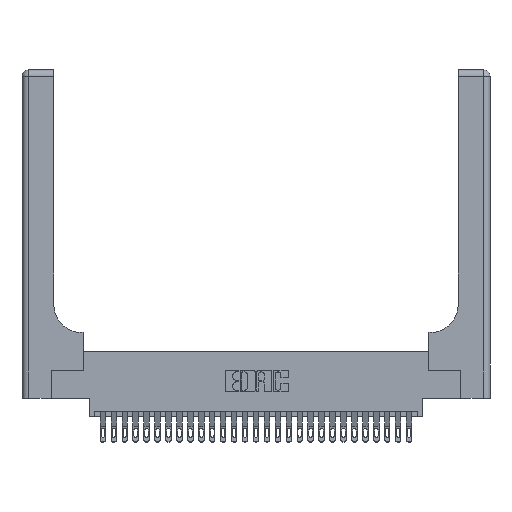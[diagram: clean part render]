
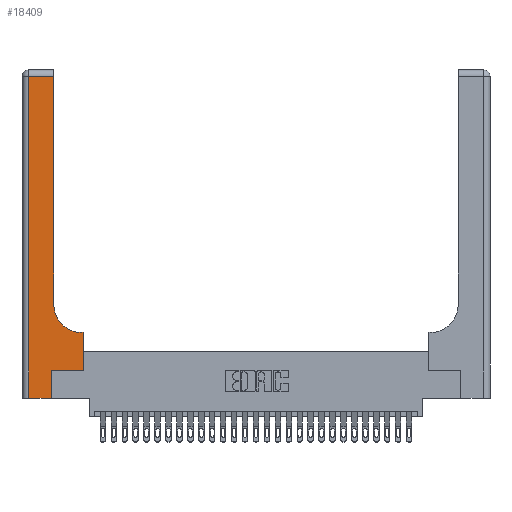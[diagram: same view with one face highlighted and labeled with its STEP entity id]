
A CAD part, top view. The second image highlights one B-rep face of the part: STEP entity #18409.
In plain terms, the highlighted planar face has unit normal (0, 0, 1).
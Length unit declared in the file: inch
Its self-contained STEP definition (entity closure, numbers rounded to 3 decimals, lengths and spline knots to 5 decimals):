
#286 = LINE ( 'NONE', #29369, #20678 ) ;
#316 = ORIENTED_EDGE ( 'NONE', *, *, #1846, .T. ) ;
#583 = LINE ( 'NONE', #9753, #21676 ) ;
#1080 = CARTESIAN_POINT ( 'NONE',  ( 0.5415, 0.6, 0.37 ) ) ;
#1422 = DIRECTION ( 'NONE',  ( 1., 0., 0. ) ) ;
#1766 = CARTESIAN_POINT ( 'NONE',  ( 0.2915, 0.85, 0.37 ) ) ;
#1846 = EDGE_CURVE ( 'NONE', #19101, #23608, #29240, .T. ) ;
#1951 = ORIENTED_EDGE ( 'NONE', *, *, #27881, .T. ) ;
#2306 = VERTEX_POINT ( 'NONE', #18966 ) ;
#2532 = DIRECTION ( 'NONE',  ( 0., 0., -1. ) ) ;
#3046 = DIRECTION ( 'NONE',  ( 0., 1., 0. ) ) ;
#3191 = VECTOR ( 'NONE', #5815, 39.37008 ) ;
#4720 = VECTOR ( 'NONE', #18654, 39.37008 ) ;
#4853 = VECTOR ( 'NONE', #23996, 39.37008 ) ;
#5710 = EDGE_CURVE ( 'NONE', #20794, #19314, #24332, .T. ) ;
#5815 = DIRECTION ( 'NONE',  ( -1., 0., 0. ) ) ;
#5923 = VERTEX_POINT ( 'NONE', #26721 ) ;
#5955 = ORIENTED_EDGE ( 'NONE', *, *, #25699, .T. ) ;
#6012 = DIRECTION ( 'NONE',  ( 0., -1., 0. ) ) ;
#6701 = CARTESIAN_POINT ( 'NONE',  ( 0., 0., 0.37 ) ) ;
#6888 = ORIENTED_EDGE ( 'NONE', *, *, #22023, .T. ) ;
#6964 = VECTOR ( 'NONE', #27529, 39.37008 ) ;
#8255 = CARTESIAN_POINT ( 'NONE',  ( 0.06, 3., 0.37 ) ) ;
#8374 = EDGE_CURVE ( 'NONE', #19314, #13760, #583, .T. ) ;
#9335 = VECTOR ( 'NONE', #27791, 39.37008 ) ;
#9753 = CARTESIAN_POINT ( 'NONE',  ( 0.2915, 3., 0.37 ) ) ;
#10920 = VERTEX_POINT ( 'NONE', #23585 ) ;
#12818 = CARTESIAN_POINT ( 'NONE',  ( 0.2915, 0.6, 0.37 ) ) ;
#13596 = LINE ( 'NONE', #8255, #25254 ) ;
#13760 = VERTEX_POINT ( 'NONE', #16475 ) ;
#13854 = VERTEX_POINT ( 'NONE', #25062 ) ;
#14559 = LINE ( 'NONE', #6701, #6964 ) ;
#16033 = ORIENTED_EDGE ( 'NONE', *, *, #28405, .T. ) ;
#16475 = CARTESIAN_POINT ( 'NONE',  ( 0.2915, 2.94, 0.37 ) ) ;
#16547 = CARTESIAN_POINT ( 'NONE',  ( 0.5585, 0.25, 0.37 ) ) ;
#16715 = ORIENTED_EDGE ( 'NONE', *, *, #5710, .T. ) ;
#17012 = FACE_OUTER_BOUND ( 'NONE', #23075, .T. ) ;
#17304 = LINE ( 'NONE', #12818, #3191 ) ;
#17725 = CARTESIAN_POINT ( 'NONE',  ( 0., 2.94, 0.37 ) ) ;
#17906 = CARTESIAN_POINT ( 'NONE',  ( 0.5415, 0.85, 0.37 ) ) ;
#18409 = ADVANCED_FACE ( 'NONE', ( #17012 ), #21567, .F. ) ;
#18654 = DIRECTION ( 'NONE',  ( 0., 1., 0. ) ) ;
#18966 = CARTESIAN_POINT ( 'NONE',  ( 0.5585, 0.6, 0.37 ) ) ;
#19101 = VERTEX_POINT ( 'NONE', #19799 ) ;
#19314 = VERTEX_POINT ( 'NONE', #1766 ) ;
#19433 = LINE ( 'NONE', #17725, #9335 ) ;
#19799 = CARTESIAN_POINT ( 'NONE',  ( 0.269, 0., 0.37 ) ) ;
#19973 = ORIENTED_EDGE ( 'NONE', *, *, #26768, .T. ) ;
#20525 = CARTESIAN_POINT ( 'NONE',  ( 0.269, 0.25, 0.37 ) ) ;
#20678 = VECTOR ( 'NONE', #1422, 39.37008 ) ;
#20794 = VERTEX_POINT ( 'NONE', #1080 ) ;
#21567 = PLANE ( 'NONE',  #28526 ) ;
#21676 = VECTOR ( 'NONE', #3046, 39.37008 ) ;
#22023 = EDGE_CURVE ( 'NONE', #10920, #13854, #13596, .T. ) ;
#23075 = EDGE_LOOP ( 'NONE', ( #25589, #26351, #6888, #16033, #316, #5955, #1951, #19973, #16715 ) ) ;
#23441 = AXIS2_PLACEMENT_3D ( 'NONE', #17906, #2532, #27057 ) ;
#23585 = CARTESIAN_POINT ( 'NONE',  ( 0.06, 2.94, 0.37 ) ) ;
#23608 = VERTEX_POINT ( 'NONE', #20525 ) ;
#23842 = CARTESIAN_POINT ( 'NONE',  ( 0., 3., 0.37 ) ) ;
#23996 = DIRECTION ( 'NONE',  ( 0., 1., 0. ) ) ;
#24332 = CIRCLE ( 'NONE', #23441, 0.25 ) ;
#25062 = CARTESIAN_POINT ( 'NONE',  ( 0.06, 0., 0.37 ) ) ;
#25254 = VECTOR ( 'NONE', #6012, 39.37008 ) ;
#25589 = ORIENTED_EDGE ( 'NONE', *, *, #8374, .T. ) ;
#25699 = EDGE_CURVE ( 'NONE', #23608, #5923, #286, .T. ) ;
#26351 = ORIENTED_EDGE ( 'NONE', *, *, #27533, .T. ) ;
#26467 = DIRECTION ( 'NONE',  ( -1., 0., 0. ) ) ;
#26721 = CARTESIAN_POINT ( 'NONE',  ( 0.5585, 0.25, 0.37 ) ) ;
#26768 = EDGE_CURVE ( 'NONE', #2306, #20794, #17304, .T. ) ;
#27057 = DIRECTION ( 'NONE',  ( 1., 0., 0. ) ) ;
#27529 = DIRECTION ( 'NONE',  ( 1., 0., 0. ) ) ;
#27533 = EDGE_CURVE ( 'NONE', #13760, #10920, #19433, .T. ) ;
#27791 = DIRECTION ( 'NONE',  ( -1., 0., 0. ) ) ;
#27881 = EDGE_CURVE ( 'NONE', #5923, #2306, #29106, .T. ) ;
#28405 = EDGE_CURVE ( 'NONE', #13854, #19101, #14559, .T. ) ;
#28526 = AXIS2_PLACEMENT_3D ( 'NONE', #23842, #28613, #26467 ) ;
#28613 = DIRECTION ( 'NONE',  ( 0., 0., -1. ) ) ;
#28666 = CARTESIAN_POINT ( 'NONE',  ( 0.269, 0., 0.37 ) ) ;
#29106 = LINE ( 'NONE', #16547, #4720 ) ;
#29240 = LINE ( 'NONE', #28666, #4853 ) ;
#29369 = CARTESIAN_POINT ( 'NONE',  ( 0.269, 0.25, 0.37 ) ) ;
